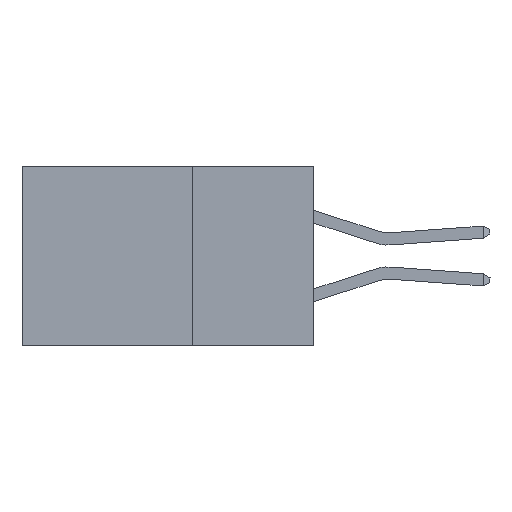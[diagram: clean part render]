
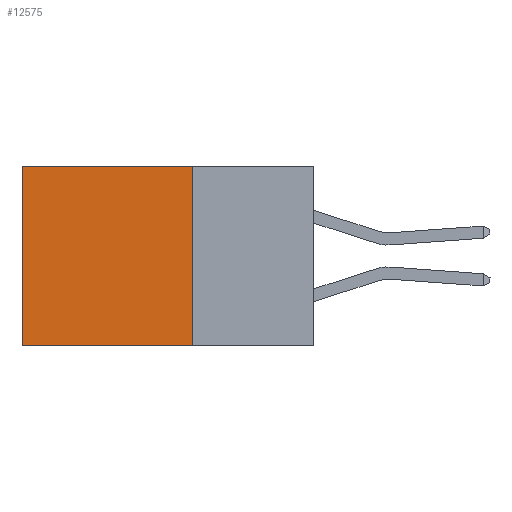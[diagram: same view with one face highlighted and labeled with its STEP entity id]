
A CAD part, left-side view. The second image highlights one B-rep face of the part: STEP entity #12575.
In plain terms, the highlighted planar face has unit normal (-1, 0, 0).
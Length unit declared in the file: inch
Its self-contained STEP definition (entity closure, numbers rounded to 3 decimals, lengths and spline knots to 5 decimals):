
#191 = VECTOR ( 'NONE', #17770, 39.37008 ) ;
#348 = EDGE_CURVE ( 'NONE', #4639, #5482, #2691, .T. ) ;
#791 = DIRECTION ( 'NONE',  ( 1., 0., 0. ) ) ;
#917 = PLANE ( 'NONE',  #16806 ) ;
#1403 = CARTESIAN_POINT ( 'NONE',  ( 0.2875, 0.6, -0.37 ) ) ;
#2116 = EDGE_CURVE ( 'NONE', #4639, #12168, #12746, .T. ) ;
#2504 = EDGE_LOOP ( 'NONE', ( #19736, #16369, #4711, #18783 ) ) ;
#2691 = LINE ( 'NONE', #6309, #21634 ) ;
#2937 = CARTESIAN_POINT ( 'NONE',  ( 0.2875, 0.25, -0.37 ) ) ;
#4639 = VERTEX_POINT ( 'NONE', #4887 ) ;
#4711 = ORIENTED_EDGE ( 'NONE', *, *, #2116, .F. ) ;
#4887 = CARTESIAN_POINT ( 'NONE',  ( 0.2875, 0.25, 0. ) ) ;
#5482 = VERTEX_POINT ( 'NONE', #5847 ) ;
#5654 = DIRECTION ( 'NONE',  ( 0., 0., -1. ) ) ;
#5847 = CARTESIAN_POINT ( 'NONE',  ( 0.2875, 0.6, 0. ) ) ;
#6191 = LINE ( 'NONE', #6317, #191 ) ;
#6309 = CARTESIAN_POINT ( 'NONE',  ( 0.2875, 0.25, 0. ) ) ;
#6317 = CARTESIAN_POINT ( 'NONE',  ( 0.2875, 0.25, -0.37 ) ) ;
#9126 = LINE ( 'NONE', #24133, #13653 ) ;
#10351 = CARTESIAN_POINT ( 'NONE',  ( 0.2875, 0.25, 0. ) ) ;
#12168 = VERTEX_POINT ( 'NONE', #2937 ) ;
#12275 = DIRECTION ( 'NONE',  ( 0., 0., -1. ) ) ;
#12387 = EDGE_CURVE ( 'NONE', #5482, #20858, #9126, .T. ) ;
#12575 = ADVANCED_FACE ( 'NONE', ( #17969 ), #917, .F. ) ;
#12746 = LINE ( 'NONE', #21614, #14665 ) ;
#13653 = VECTOR ( 'NONE', #5654, 39.37008 ) ;
#13931 = DIRECTION ( 'NONE',  ( 0., 0., -1. ) ) ;
#14665 = VECTOR ( 'NONE', #12275, 39.37008 ) ;
#16369 = ORIENTED_EDGE ( 'NONE', *, *, #18970, .F. ) ;
#16806 = AXIS2_PLACEMENT_3D ( 'NONE', #10351, #791, #13931 ) ;
#17770 = DIRECTION ( 'NONE',  ( 0., 1., 0. ) ) ;
#17969 = FACE_OUTER_BOUND ( 'NONE', #2504, .T. ) ;
#18783 = ORIENTED_EDGE ( 'NONE', *, *, #348, .T. ) ;
#18970 = EDGE_CURVE ( 'NONE', #12168, #20858, #6191, .T. ) ;
#19736 = ORIENTED_EDGE ( 'NONE', *, *, #12387, .T. ) ;
#20858 = VERTEX_POINT ( 'NONE', #1403 ) ;
#21614 = CARTESIAN_POINT ( 'NONE',  ( 0.2875, 0.25, 0. ) ) ;
#21634 = VECTOR ( 'NONE', #23191, 39.37008 ) ;
#23191 = DIRECTION ( 'NONE',  ( 0., 1., 0. ) ) ;
#24133 = CARTESIAN_POINT ( 'NONE',  ( 0.2875, 0.6, 0. ) ) ;
